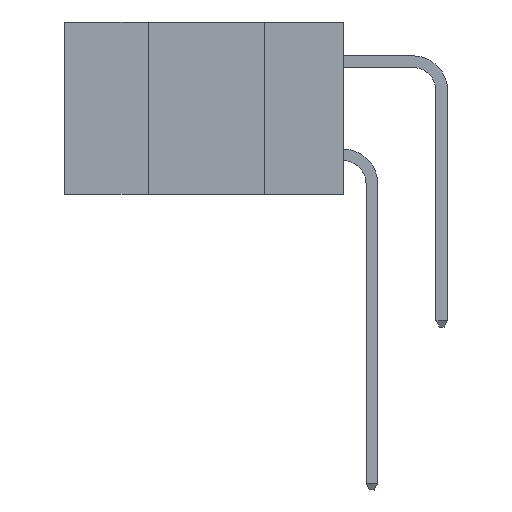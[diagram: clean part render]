
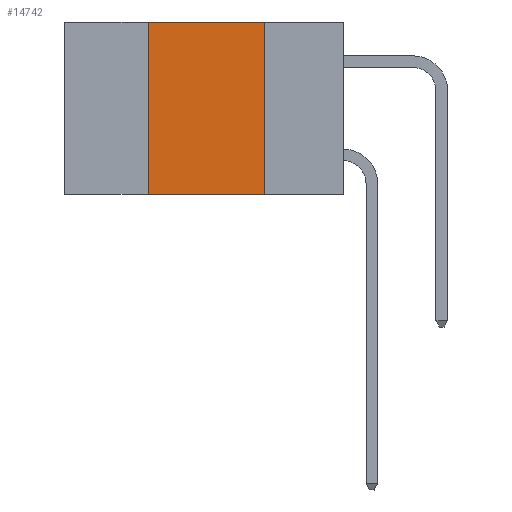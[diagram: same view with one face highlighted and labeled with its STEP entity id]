
A CAD part, left-side view. The second image highlights one B-rep face of the part: STEP entity #14742.
In plain terms, the highlighted planar face has unit normal (-1, 0, 0).
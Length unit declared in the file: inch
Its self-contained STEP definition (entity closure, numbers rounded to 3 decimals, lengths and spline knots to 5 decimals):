
#319 = CARTESIAN_POINT ( 'NONE',  ( 0., 0.42, 0. ) ) ;
#585 = VERTEX_POINT ( 'NONE', #5272 ) ;
#639 = CARTESIAN_POINT ( 'NONE',  ( 0., 0.6, 0. ) ) ;
#827 = CARTESIAN_POINT ( 'NONE',  ( 0., 0.6, 0. ) ) ;
#1164 = FACE_OUTER_BOUND ( 'NONE', #4269, .T. ) ;
#2339 = DIRECTION ( 'NONE',  ( 0., 0., -1. ) ) ;
#2379 = VERTEX_POINT ( 'NONE', #6826 ) ;
#2768 = ORIENTED_EDGE ( 'NONE', *, *, #11698, .F. ) ;
#2912 = CARTESIAN_POINT ( 'NONE',  ( 0., 0.42, -0.37 ) ) ;
#2919 = VECTOR ( 'NONE', #12105, 39.37008 ) ;
#4020 = CARTESIAN_POINT ( 'NONE',  ( 0., 0.42, 0. ) ) ;
#4149 = CARTESIAN_POINT ( 'NONE',  ( 0., 0.6, -0.37 ) ) ;
#4269 = EDGE_LOOP ( 'NONE', ( #15283, #2768, #10613, #4608 ) ) ;
#4608 = ORIENTED_EDGE ( 'NONE', *, *, #15583, .T. ) ;
#5272 = CARTESIAN_POINT ( 'NONE',  ( 0., 0.17, 0. ) ) ;
#5582 = VERTEX_POINT ( 'NONE', #319 ) ;
#6749 = LINE ( 'NONE', #639, #2919 ) ;
#6826 = CARTESIAN_POINT ( 'NONE',  ( 0., 0.17, -0.37 ) ) ;
#7220 = DIRECTION ( 'NONE',  ( 0., 0., -1. ) ) ;
#7801 = DIRECTION ( 'NONE',  ( 0., 0., 1. ) ) ;
#7828 = VECTOR ( 'NONE', #7801, 39.37008 ) ;
#7993 = DIRECTION ( 'NONE',  ( 0., -1., 0. ) ) ;
#8159 = LINE ( 'NONE', #4149, #14461 ) ;
#8325 = AXIS2_PLACEMENT_3D ( 'NONE', #827, #14795, #7220 ) ;
#8424 = EDGE_CURVE ( 'NONE', #16252, #5582, #14149, .T. ) ;
#9552 = VECTOR ( 'NONE', #2339, 39.37008 ) ;
#10613 = ORIENTED_EDGE ( 'NONE', *, *, #8424, .F. ) ;
#11698 = EDGE_CURVE ( 'NONE', #5582, #585, #6749, .T. ) ;
#11945 = EDGE_CURVE ( 'NONE', #585, #2379, #13296, .T. ) ;
#12105 = DIRECTION ( 'NONE',  ( 0., -1., 0. ) ) ;
#12297 = PLANE ( 'NONE',  #8325 ) ;
#12531 = CARTESIAN_POINT ( 'NONE',  ( 0., 0.17, 0. ) ) ;
#13296 = LINE ( 'NONE', #12531, #9552 ) ;
#14149 = LINE ( 'NONE', #4020, #7828 ) ;
#14461 = VECTOR ( 'NONE', #7993, 39.37008 ) ;
#14742 = ADVANCED_FACE ( 'NONE', ( #1164 ), #12297, .F. ) ;
#14795 = DIRECTION ( 'NONE',  ( 1., 0., 0. ) ) ;
#15283 = ORIENTED_EDGE ( 'NONE', *, *, #11945, .F. ) ;
#15583 = EDGE_CURVE ( 'NONE', #16252, #2379, #8159, .T. ) ;
#16252 = VERTEX_POINT ( 'NONE', #2912 ) ;
